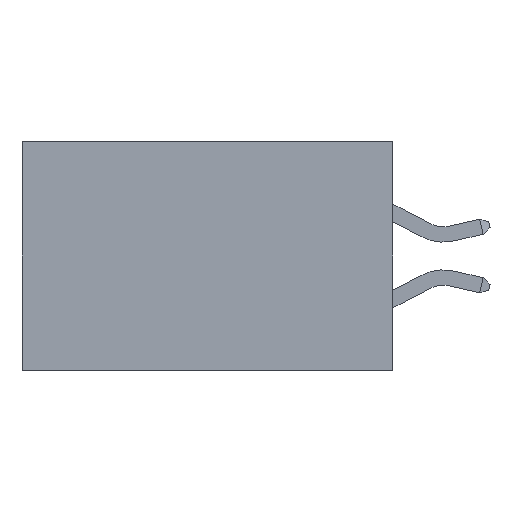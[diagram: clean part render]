
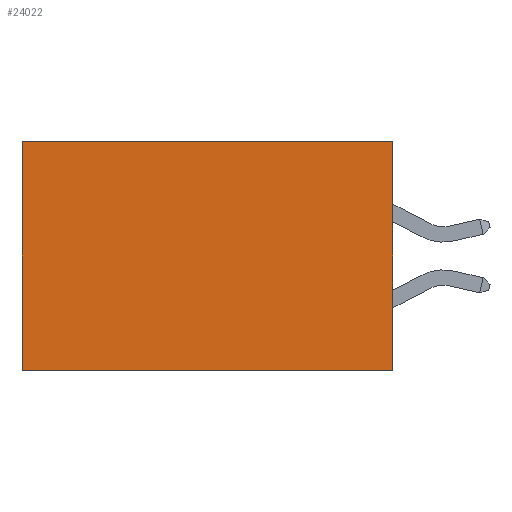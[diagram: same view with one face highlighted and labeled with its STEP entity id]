
A CAD part, left-side view. The second image highlights one B-rep face of the part: STEP entity #24022.
In plain terms, the highlighted planar face has unit normal (-1, 0, 0).
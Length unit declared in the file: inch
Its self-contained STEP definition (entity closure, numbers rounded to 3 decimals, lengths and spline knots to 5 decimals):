
#3284 = ORIENTED_EDGE ( 'NONE', *, *, #37041, .F. ) ;
#3535 = DIRECTION ( 'NONE',  ( 0., 0., -1. ) ) ;
#4080 = CARTESIAN_POINT ( 'NONE',  ( 0.2875, 0., 0. ) ) ;
#4686 = EDGE_CURVE ( 'NONE', #33352, #15929, #13290, .T. ) ;
#5864 = VERTEX_POINT ( 'NONE', #38756 ) ;
#7604 = LINE ( 'NONE', #27675, #17158 ) ;
#7614 = ORIENTED_EDGE ( 'NONE', *, *, #13592, .F. ) ;
#7636 = AXIS2_PLACEMENT_3D ( 'NONE', #4080, #25526, #10181 ) ;
#9088 = VECTOR ( 'NONE', #31594, 39.37008 ) ;
#9897 = CARTESIAN_POINT ( 'NONE',  ( 0.2875, 0., 0. ) ) ;
#10181 = DIRECTION ( 'NONE',  ( 0., 0., -1. ) ) ;
#11201 = CARTESIAN_POINT ( 'NONE',  ( 0.2875, 0.6, -0.37 ) ) ;
#13290 = LINE ( 'NONE', #13681, #26304 ) ;
#13487 = ORIENTED_EDGE ( 'NONE', *, *, #22660, .T. ) ;
#13592 = EDGE_CURVE ( 'NONE', #35523, #15929, #24011, .T. ) ;
#13681 = CARTESIAN_POINT ( 'NONE',  ( 0.2875, 0.6, 0. ) ) ;
#13841 = CARTESIAN_POINT ( 'NONE',  ( 0.2875, 0., -0.37 ) ) ;
#13938 = LINE ( 'NONE', #9897, #9088 ) ;
#15929 = VERTEX_POINT ( 'NONE', #11201 ) ;
#16789 = DIRECTION ( 'NONE',  ( 0., 0., -1. ) ) ;
#17158 = VECTOR ( 'NONE', #3535, 39.37008 ) ;
#22660 = EDGE_CURVE ( 'NONE', #5864, #33352, #13938, .T. ) ;
#24011 = LINE ( 'NONE', #32426, #39183 ) ;
#24022 = ADVANCED_FACE ( 'NONE', ( #24910 ), #37873, .F. ) ;
#24910 = FACE_OUTER_BOUND ( 'NONE', #36058, .T. ) ;
#25526 = DIRECTION ( 'NONE',  ( 1., 0., 0. ) ) ;
#26281 = ORIENTED_EDGE ( 'NONE', *, *, #4686, .T. ) ;
#26304 = VECTOR ( 'NONE', #16789, 39.37008 ) ;
#27675 = CARTESIAN_POINT ( 'NONE',  ( 0.2875, 0., 0. ) ) ;
#31594 = DIRECTION ( 'NONE',  ( 0., 1., 0. ) ) ;
#32426 = CARTESIAN_POINT ( 'NONE',  ( 0.2875, 0., -0.37 ) ) ;
#33352 = VERTEX_POINT ( 'NONE', #35180 ) ;
#34186 = DIRECTION ( 'NONE',  ( 0., 1., 0. ) ) ;
#35180 = CARTESIAN_POINT ( 'NONE',  ( 0.2875, 0.6, 0. ) ) ;
#35523 = VERTEX_POINT ( 'NONE', #13841 ) ;
#36058 = EDGE_LOOP ( 'NONE', ( #26281, #7614, #3284, #13487 ) ) ;
#37041 = EDGE_CURVE ( 'NONE', #5864, #35523, #7604, .T. ) ;
#37873 = PLANE ( 'NONE',  #7636 ) ;
#38756 = CARTESIAN_POINT ( 'NONE',  ( 0.2875, 0., 0. ) ) ;
#39183 = VECTOR ( 'NONE', #34186, 39.37008 ) ;
